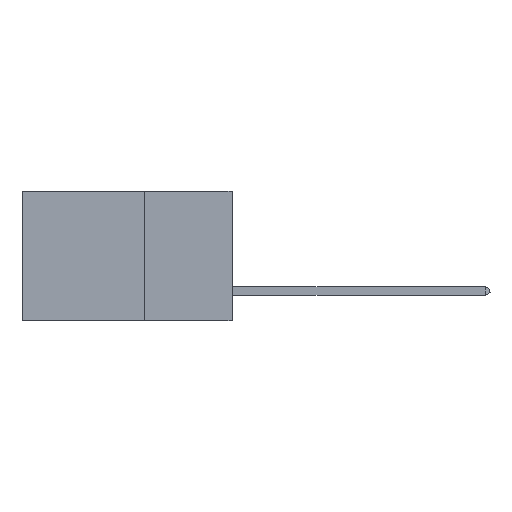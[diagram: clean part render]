
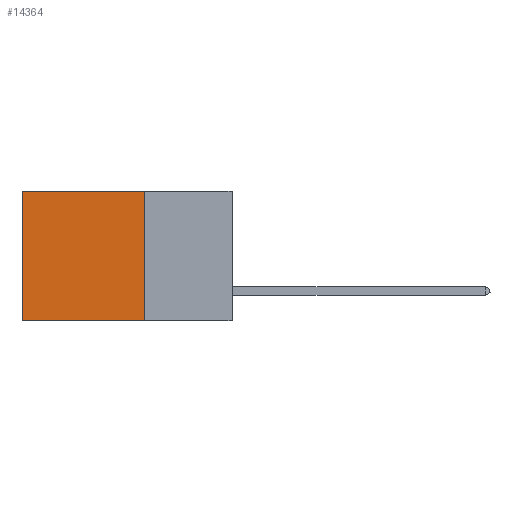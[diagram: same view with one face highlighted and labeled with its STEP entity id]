
A CAD part, left-side view. The second image highlights one B-rep face of the part: STEP entity #14364.
In plain terms, the highlighted planar face has unit normal (-1, 0, 0).
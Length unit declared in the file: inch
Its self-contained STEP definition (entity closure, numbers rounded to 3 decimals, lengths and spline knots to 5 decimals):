
#764 = AXIS2_PLACEMENT_3D ( 'NONE', #5970, #13460, #9438 ) ;
#1010 = EDGE_CURVE ( 'NONE', #10234, #14611, #6834, .T. ) ;
#1281 = FACE_OUTER_BOUND ( 'NONE', #5847, .T. ) ;
#2446 = CARTESIAN_POINT ( 'NONE',  ( 0.2875, 0.25, 0. ) ) ;
#2866 = VECTOR ( 'NONE', #14404, 39.37008 ) ;
#3319 = DIRECTION ( 'NONE',  ( 0., 1., 0. ) ) ;
#3392 = ORIENTED_EDGE ( 'NONE', *, *, #7951, .T. ) ;
#5431 = ORIENTED_EDGE ( 'NONE', *, *, #8848, .T. ) ;
#5554 = VECTOR ( 'NONE', #13689, 39.37008 ) ;
#5847 = EDGE_LOOP ( 'NONE', ( #3392, #12494, #16543, #5431 ) ) ;
#5970 = CARTESIAN_POINT ( 'NONE',  ( 0.2875, 0.25, 0. ) ) ;
#6834 = LINE ( 'NONE', #2446, #2866 ) ;
#6970 = CARTESIAN_POINT ( 'NONE',  ( 0.2875, 0.25, 0. ) ) ;
#7587 = CARTESIAN_POINT ( 'NONE',  ( 0.2875, 0.6, 0. ) ) ;
#7668 = PLANE ( 'NONE',  #764 ) ;
#7951 = EDGE_CURVE ( 'NONE', #16915, #10627, #13583, .T. ) ;
#8137 = CARTESIAN_POINT ( 'NONE',  ( 0.2875, 0.6, 0. ) ) ;
#8252 = CARTESIAN_POINT ( 'NONE',  ( 0.2875, 0.6, -0.37 ) ) ;
#8687 = VECTOR ( 'NONE', #3319, 39.37008 ) ;
#8848 = EDGE_CURVE ( 'NONE', #10234, #16915, #13408, .T. ) ;
#9071 = CARTESIAN_POINT ( 'NONE',  ( 0.2875, 0.25, -0.37 ) ) ;
#9087 = DIRECTION ( 'NONE',  ( 0., 0., -1. ) ) ;
#9438 = DIRECTION ( 'NONE',  ( 0., 0., -1. ) ) ;
#9593 = VECTOR ( 'NONE', #9087, 39.37008 ) ;
#9616 = CARTESIAN_POINT ( 'NONE',  ( 0.2875, 0.25, -0.37 ) ) ;
#10234 = VERTEX_POINT ( 'NONE', #6970 ) ;
#10627 = VERTEX_POINT ( 'NONE', #8252 ) ;
#10876 = LINE ( 'NONE', #9071, #5554 ) ;
#12494 = ORIENTED_EDGE ( 'NONE', *, *, #17918, .F. ) ;
#13408 = LINE ( 'NONE', #15126, #8687 ) ;
#13460 = DIRECTION ( 'NONE',  ( 1., 0., 0. ) ) ;
#13583 = LINE ( 'NONE', #7587, #9593 ) ;
#13689 = DIRECTION ( 'NONE',  ( 0., 1., 0. ) ) ;
#14364 = ADVANCED_FACE ( 'NONE', ( #1281 ), #7668, .F. ) ;
#14404 = DIRECTION ( 'NONE',  ( 0., 0., -1. ) ) ;
#14611 = VERTEX_POINT ( 'NONE', #9616 ) ;
#15126 = CARTESIAN_POINT ( 'NONE',  ( 0.2875, 0.25, 0. ) ) ;
#16543 = ORIENTED_EDGE ( 'NONE', *, *, #1010, .F. ) ;
#16915 = VERTEX_POINT ( 'NONE', #8137 ) ;
#17918 = EDGE_CURVE ( 'NONE', #14611, #10627, #10876, .T. ) ;
